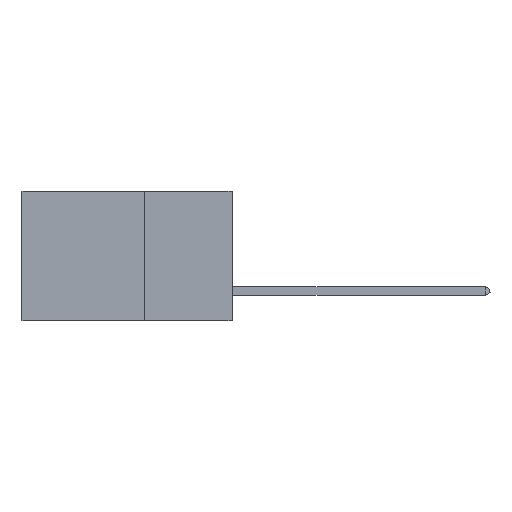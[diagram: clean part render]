
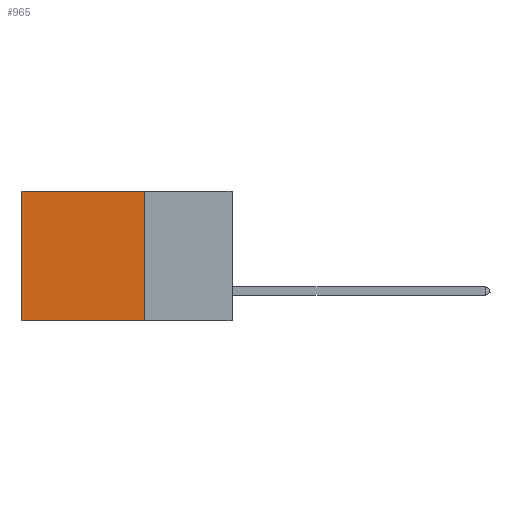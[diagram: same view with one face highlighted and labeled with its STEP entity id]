
A CAD part, left-side view. The second image highlights one B-rep face of the part: STEP entity #965.
In plain terms, the highlighted planar face has unit normal (-1, 0, 0).
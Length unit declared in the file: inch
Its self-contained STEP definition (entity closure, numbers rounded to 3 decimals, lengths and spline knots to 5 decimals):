
#850 = VERTEX_POINT ( 'NONE', #18112 ) ;
#965 = ADVANCED_FACE ( 'NONE', ( #14858 ), #14180, .F. ) ;
#1255 = EDGE_CURVE ( 'NONE', #850, #18882, #2771, .T. ) ;
#1742 = LINE ( 'NONE', #4212, #21864 ) ;
#2080 = VECTOR ( 'NONE', #19500, 39.37008 ) ;
#2714 = ORIENTED_EDGE ( 'NONE', *, *, #22969, .T. ) ;
#2771 = LINE ( 'NONE', #19604, #2080 ) ;
#4212 = CARTESIAN_POINT ( 'NONE',  ( 0.2875, 0.25, 0. ) ) ;
#5489 = CARTESIAN_POINT ( 'NONE',  ( 0.2875, 0.25, -0.37 ) ) ;
#10962 = AXIS2_PLACEMENT_3D ( 'NONE', #21886, #23248, #25296 ) ;
#11140 = EDGE_CURVE ( 'NONE', #23255, #27035, #11807, .T. ) ;
#11271 = DIRECTION ( 'NONE',  ( 0., 1., 0. ) ) ;
#11807 = LINE ( 'NONE', #30144, #24698 ) ;
#12008 = DIRECTION ( 'NONE',  ( 0., 1., 0. ) ) ;
#12359 = VECTOR ( 'NONE', #12008, 39.37008 ) ;
#13835 = LINE ( 'NONE', #21329, #12359 ) ;
#14180 = PLANE ( 'NONE',  #10962 ) ;
#14510 = EDGE_CURVE ( 'NONE', #18882, #27035, #13835, .T. ) ;
#14858 = FACE_OUTER_BOUND ( 'NONE', #17312, .T. ) ;
#15786 = DIRECTION ( 'NONE',  ( 0., 0., -1. ) ) ;
#16767 = ORIENTED_EDGE ( 'NONE', *, *, #1255, .F. ) ;
#17312 = EDGE_LOOP ( 'NONE', ( #21789, #27805, #16767, #2714 ) ) ;
#18112 = CARTESIAN_POINT ( 'NONE',  ( 0.2875, 0.25, 0. ) ) ;
#18882 = VERTEX_POINT ( 'NONE', #5489 ) ;
#19037 = CARTESIAN_POINT ( 'NONE',  ( 0.2875, 0.6, 0. ) ) ;
#19500 = DIRECTION ( 'NONE',  ( 0., 0., -1. ) ) ;
#19604 = CARTESIAN_POINT ( 'NONE',  ( 0.2875, 0.25, 0. ) ) ;
#21329 = CARTESIAN_POINT ( 'NONE',  ( 0.2875, 0.25, -0.37 ) ) ;
#21789 = ORIENTED_EDGE ( 'NONE', *, *, #11140, .T. ) ;
#21864 = VECTOR ( 'NONE', #11271, 39.37008 ) ;
#21886 = CARTESIAN_POINT ( 'NONE',  ( 0.2875, 0.25, 0. ) ) ;
#22969 = EDGE_CURVE ( 'NONE', #850, #23255, #1742, .T. ) ;
#23248 = DIRECTION ( 'NONE',  ( 1., 0., 0. ) ) ;
#23255 = VERTEX_POINT ( 'NONE', #19037 ) ;
#24698 = VECTOR ( 'NONE', #15786, 39.37008 ) ;
#25296 = DIRECTION ( 'NONE',  ( 0., 0., -1. ) ) ;
#27035 = VERTEX_POINT ( 'NONE', #28965 ) ;
#27805 = ORIENTED_EDGE ( 'NONE', *, *, #14510, .F. ) ;
#28965 = CARTESIAN_POINT ( 'NONE',  ( 0.2875, 0.6, -0.37 ) ) ;
#30144 = CARTESIAN_POINT ( 'NONE',  ( 0.2875, 0.6, 0. ) ) ;
